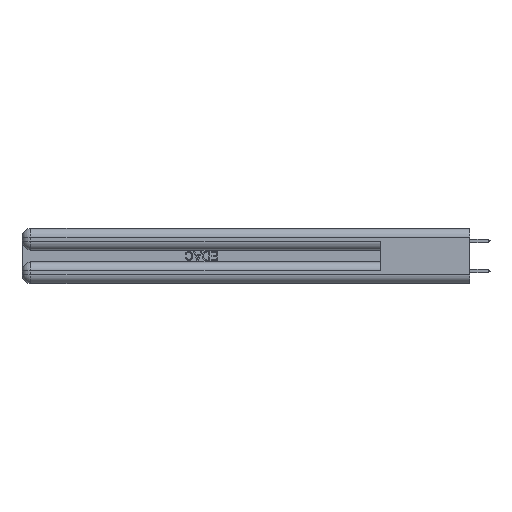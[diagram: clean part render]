
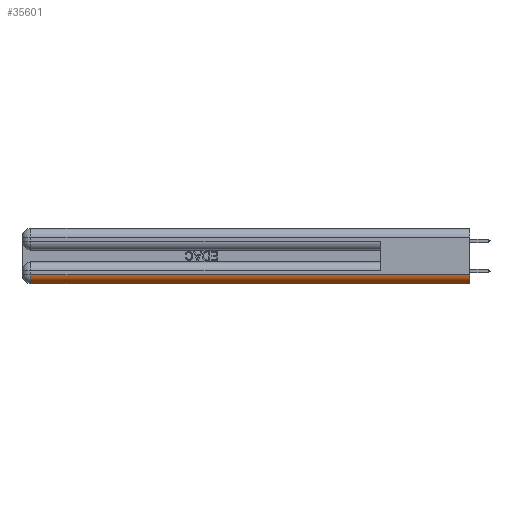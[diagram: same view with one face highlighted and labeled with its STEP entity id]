
A CAD part, left-side view. The second image highlights one B-rep face of the part: STEP entity #35601.
In plain terms, the highlighted cylindrical face has radius 1.524 mm (diameter 3.048 mm), a partial arc.
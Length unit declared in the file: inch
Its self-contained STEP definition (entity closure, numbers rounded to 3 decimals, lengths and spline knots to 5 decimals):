
#2163 = VERTEX_POINT ( 'NONE', #18705 ) ;
#2536 = CARTESIAN_POINT ( 'NONE',  ( 0.06, 0., 0.06 ) ) ;
#2573 = VERTEX_POINT ( 'NONE', #11136 ) ;
#4914 = EDGE_CURVE ( 'NONE', #2573, #15370, #30048, .T. ) ;
#7622 = CARTESIAN_POINT ( 'NONE',  ( 0.06, 3., 0. ) ) ;
#7894 = DIRECTION ( 'NONE',  ( 0., 1., 0. ) ) ;
#9264 = DIRECTION ( 'NONE',  ( 0., -1., 0. ) ) ;
#9768 = EDGE_LOOP ( 'NONE', ( #39627, #12666, #11344, #17771 ) ) ;
#10440 = CARTESIAN_POINT ( 'NONE',  ( 0.06, 2.94, 0. ) ) ;
#11136 = CARTESIAN_POINT ( 'NONE',  ( 0.06, 0., 0. ) ) ;
#11344 = ORIENTED_EDGE ( 'NONE', *, *, #22775, .F. ) ;
#11896 = CIRCLE ( 'NONE', #39411, 0.06 ) ;
#12323 = VECTOR ( 'NONE', #7894, 39.37008 ) ;
#12369 = VECTOR ( 'NONE', #19082, 39.37008 ) ;
#12666 = ORIENTED_EDGE ( 'NONE', *, *, #22886, .F. ) ;
#12765 = CARTESIAN_POINT ( 'NONE',  ( 0., 0., 0.06 ) ) ;
#15159 = DIRECTION ( 'NONE',  ( 0., 1., 0. ) ) ;
#15370 = VERTEX_POINT ( 'NONE', #10440 ) ;
#16210 = CYLINDRICAL_SURFACE ( 'NONE', #40678, 0.06 ) ;
#16436 = AXIS2_PLACEMENT_3D ( 'NONE', #28126, #9264, #31260 ) ;
#17771 = ORIENTED_EDGE ( 'NONE', *, *, #4914, .F. ) ;
#18329 = DIRECTION ( 'NONE',  ( 0., 0., 1. ) ) ;
#18384 = DIRECTION ( 'NONE',  ( 0., 1., 0. ) ) ;
#18705 = CARTESIAN_POINT ( 'NONE',  ( 0., 0., 0.06 ) ) ;
#18911 = CARTESIAN_POINT ( 'NONE',  ( 0., 2.94, 0.06 ) ) ;
#19082 = DIRECTION ( 'NONE',  ( 0., -1., 0. ) ) ;
#21617 = EDGE_CURVE ( 'NONE', #2163, #2573, #35496, .T. ) ;
#22775 = EDGE_CURVE ( 'NONE', #15370, #23982, #11896, .T. ) ;
#22886 = EDGE_CURVE ( 'NONE', #23982, #2163, #37491, .T. ) ;
#23982 = VERTEX_POINT ( 'NONE', #18911 ) ;
#24567 = FACE_OUTER_BOUND ( 'NONE', #9768, .T. ) ;
#28126 = CARTESIAN_POINT ( 'NONE',  ( 0.06, 0., 0.06 ) ) ;
#30048 = LINE ( 'NONE', #7622, #12323 ) ;
#31260 = DIRECTION ( 'NONE',  ( 0., 0., 1. ) ) ;
#35496 = CIRCLE ( 'NONE', #16436, 0.06 ) ;
#35601 = ADVANCED_FACE ( 'NONE', ( #24567 ), #16210, .T. ) ;
#37267 = CARTESIAN_POINT ( 'NONE',  ( 0.06, 2.94, 0.06 ) ) ;
#37491 = LINE ( 'NONE', #12765, #12369 ) ;
#39411 = AXIS2_PLACEMENT_3D ( 'NONE', #37267, #18384, #40402 ) ;
#39627 = ORIENTED_EDGE ( 'NONE', *, *, #21617, .F. ) ;
#40402 = DIRECTION ( 'NONE',  ( 0., 0., 1. ) ) ;
#40678 = AXIS2_PLACEMENT_3D ( 'NONE', #2536, #15159, #18329 ) ;
